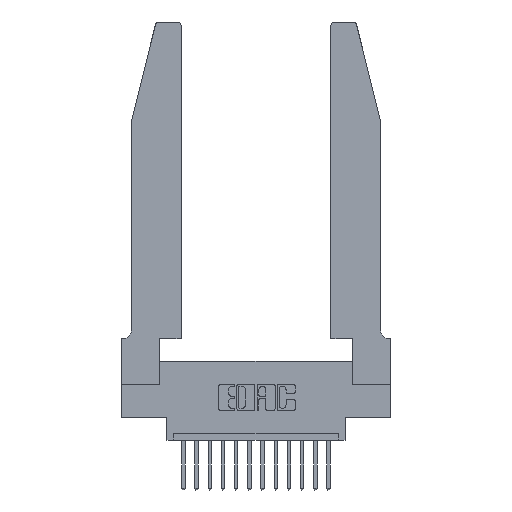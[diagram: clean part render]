
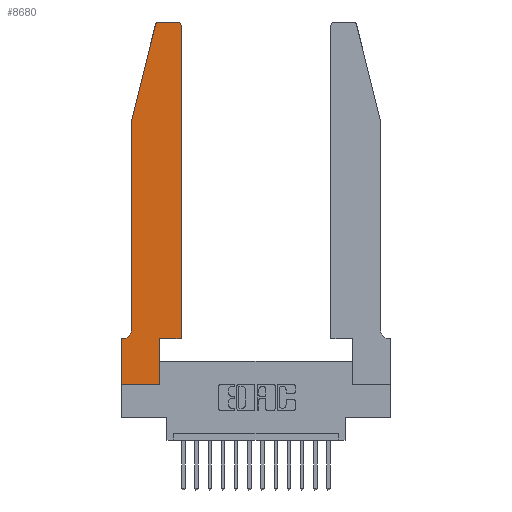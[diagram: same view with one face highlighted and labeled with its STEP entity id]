
A CAD part, top view. The second image highlights one B-rep face of the part: STEP entity #8680.
In plain terms, the highlighted planar face has unit normal (0, 0, 1).
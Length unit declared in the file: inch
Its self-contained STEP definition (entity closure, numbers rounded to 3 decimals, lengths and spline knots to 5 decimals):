
#162 = CARTESIAN_POINT ( 'NONE',  ( 0.0755, 2., 0.37 ) ) ;
#264 = VERTEX_POINT ( 'NONE', #16240 ) ;
#308 = VERTEX_POINT ( 'NONE', #8545 ) ;
#550 = ORIENTED_EDGE ( 'NONE', *, *, #2404, .T. ) ;
#979 = ORIENTED_EDGE ( 'NONE', *, *, #16185, .T. ) ;
#1325 = ORIENTED_EDGE ( 'NONE', *, *, #13754, .T. ) ;
#1422 = EDGE_CURVE ( 'NONE', #3735, #16427, #5521, .T. ) ;
#1451 = ORIENTED_EDGE ( 'NONE', *, *, #1422, .T. ) ;
#1452 = EDGE_CURVE ( 'NONE', #264, #11926, #15490, .T. ) ;
#1501 = CARTESIAN_POINT ( 'NONE',  ( 0.2865, 0.35, 0.37 ) ) ;
#2404 = EDGE_CURVE ( 'NONE', #3888, #9783, #6743, .T. ) ;
#2484 = ORIENTED_EDGE ( 'NONE', *, *, #10499, .T. ) ;
#2509 = LINE ( 'NONE', #3486, #11164 ) ;
#2573 = LINE ( 'NONE', #11310, #11211 ) ;
#2923 = FACE_OUTER_BOUND ( 'NONE', #5593, .T. ) ;
#3100 = EDGE_CURVE ( 'NONE', #11926, #308, #15643, .T. ) ;
#3486 = CARTESIAN_POINT ( 'NONE',  ( 0.4505, 0.35, 0.37 ) ) ;
#3735 = VERTEX_POINT ( 'NONE', #7786 ) ;
#3888 = VERTEX_POINT ( 'NONE', #14912 ) ;
#4211 = DIRECTION ( 'NONE',  ( 0., 1., 0. ) ) ;
#4612 = CARTESIAN_POINT ( 'NONE',  ( 0.284, 2.72, 0.37 ) ) ;
#4702 = AXIS2_PLACEMENT_3D ( 'NONE', #14642, #4958, #8981 ) ;
#4728 = DIRECTION ( 'NONE',  ( 0., 0., 1. ) ) ;
#4818 = VECTOR ( 'NONE', #17328, 39.37008 ) ;
#4958 = DIRECTION ( 'NONE',  ( 0., 0., 1. ) ) ;
#5153 = ORIENTED_EDGE ( 'NONE', *, *, #14551, .T. ) ;
#5156 = VECTOR ( 'NONE', #14626, 39.37008 ) ;
#5386 = DIRECTION ( 'NONE',  ( 0., 1., 0. ) ) ;
#5521 = CIRCLE ( 'NONE', #15368, 0.07 ) ;
#5593 = EDGE_LOOP ( 'NONE', ( #14481, #550, #979, #6981, #1451, #1325, #8827, #8383, #16617, #17822, #2484, #5153 ) ) ;
#5652 = DIRECTION ( 'NONE',  ( -0.239, -0.971, 0. ) ) ;
#6368 = EDGE_CURVE ( 'NONE', #11910, #3888, #15338, .T. ) ;
#6524 = LINE ( 'NONE', #162, #13690 ) ;
#6528 = VERTEX_POINT ( 'NONE', #7620 ) ;
#6743 = CIRCLE ( 'NONE', #10587, 0.03 ) ;
#6981 = ORIENTED_EDGE ( 'NONE', *, *, #10086, .T. ) ;
#7280 = VECTOR ( 'NONE', #5652, 39.37008 ) ;
#7620 = CARTESIAN_POINT ( 'NONE',  ( 0.4505, 0.35, 0.37 ) ) ;
#7624 = EDGE_CURVE ( 'NONE', #9199, #6528, #2509, .T. ) ;
#7756 = CARTESIAN_POINT ( 'NONE',  ( 0.2605, 2.75, 0.37 ) ) ;
#7786 = CARTESIAN_POINT ( 'NONE',  ( 0.0755, 0.42, 0.37 ) ) ;
#7881 = VECTOR ( 'NONE', #5386, 39.37008 ) ;
#7980 = VERTEX_POINT ( 'NONE', #9701 ) ;
#8259 = CARTESIAN_POINT ( 'NONE',  ( 0., 0., 0.37 ) ) ;
#8383 = ORIENTED_EDGE ( 'NONE', *, *, #3100, .T. ) ;
#8545 = CARTESIAN_POINT ( 'NONE',  ( 0.2865, 0., 0.37 ) ) ;
#8680 = ADVANCED_FACE ( 'NONE', ( #2923 ), #17317, .T. ) ;
#8827 = ORIENTED_EDGE ( 'NONE', *, *, #1452, .T. ) ;
#8897 = VERTEX_POINT ( 'NONE', #13616 ) ;
#8981 = DIRECTION ( 'NONE',  ( 1., 0., 0. ) ) ;
#9169 = LINE ( 'NONE', #16476, #7881 ) ;
#9199 = VERTEX_POINT ( 'NONE', #1501 ) ;
#9495 = CIRCLE ( 'NONE', #4702, 0.03 ) ;
#9701 = CARTESIAN_POINT ( 'NONE',  ( 0.4505, 2.72, 0.37 ) ) ;
#9712 = CARTESIAN_POINT ( 'NONE',  ( 0.0755, 2., 0.37 ) ) ;
#9753 = DIRECTION ( 'NONE',  ( -1., 0., 0. ) ) ;
#9783 = VERTEX_POINT ( 'NONE', #9856 ) ;
#9856 = CARTESIAN_POINT ( 'NONE',  ( 0.25487, 2.72718, 0.37 ) ) ;
#10086 = EDGE_CURVE ( 'NONE', #8897, #3735, #6524, .T. ) ;
#10265 = CARTESIAN_POINT ( 'NONE',  ( 0.0055, 0.35, 0.37 ) ) ;
#10380 = CARTESIAN_POINT ( 'NONE',  ( 0., 0., 0.37 ) ) ;
#10499 = EDGE_CURVE ( 'NONE', #6528, #7980, #9169, .T. ) ;
#10552 = AXIS2_PLACEMENT_3D ( 'NONE', #16009, #17997, #16654 ) ;
#10587 = AXIS2_PLACEMENT_3D ( 'NONE', #4612, #4728, #15564 ) ;
#10719 = CARTESIAN_POINT ( 'NONE',  ( 0., 0., 0.37 ) ) ;
#11164 = VECTOR ( 'NONE', #13161, 39.37008 ) ;
#11211 = VECTOR ( 'NONE', #4211, 39.37008 ) ;
#11239 = LINE ( 'NONE', #17971, #17152 ) ;
#11310 = CARTESIAN_POINT ( 'NONE',  ( 0.2865, 0.35, 0.37 ) ) ;
#11381 = DIRECTION ( 'NONE',  ( 0., -1., 0. ) ) ;
#11910 = VERTEX_POINT ( 'NONE', #15789 ) ;
#11926 = VERTEX_POINT ( 'NONE', #10719 ) ;
#12294 = DIRECTION ( 'NONE',  ( -1., 0., 0. ) ) ;
#12614 = DIRECTION ( 'NONE',  ( 0., 0., -1. ) ) ;
#13161 = DIRECTION ( 'NONE',  ( 1., 0., 0. ) ) ;
#13616 = CARTESIAN_POINT ( 'NONE',  ( 0.0755, 2., 0.37 ) ) ;
#13690 = VECTOR ( 'NONE', #15449, 39.37008 ) ;
#13754 = EDGE_CURVE ( 'NONE', #16427, #264, #11239, .T. ) ;
#14481 = ORIENTED_EDGE ( 'NONE', *, *, #6368, .T. ) ;
#14551 = EDGE_CURVE ( 'NONE', #7980, #11910, #9495, .T. ) ;
#14626 = DIRECTION ( 'NONE',  ( -1., 0., 0. ) ) ;
#14642 = CARTESIAN_POINT ( 'NONE',  ( 0.4205, 2.72, 0.37 ) ) ;
#14880 = CARTESIAN_POINT ( 'NONE',  ( 0.0055, 0.42, 0.37 ) ) ;
#14912 = CARTESIAN_POINT ( 'NONE',  ( 0.284, 2.75, 0.37 ) ) ;
#14986 = EDGE_CURVE ( 'NONE', #308, #9199, #2573, .T. ) ;
#15338 = LINE ( 'NONE', #7756, #5156 ) ;
#15368 = AXIS2_PLACEMENT_3D ( 'NONE', #14880, #12614, #9753 ) ;
#15449 = DIRECTION ( 'NONE',  ( 0., -1., 0. ) ) ;
#15490 = LINE ( 'NONE', #8259, #16806 ) ;
#15564 = DIRECTION ( 'NONE',  ( 1., 0., 0. ) ) ;
#15643 = LINE ( 'NONE', #10380, #4818 ) ;
#15789 = CARTESIAN_POINT ( 'NONE',  ( 0.4205, 2.75, 0.37 ) ) ;
#16009 = CARTESIAN_POINT ( 'NONE',  ( 0., 0.35, 0.37 ) ) ;
#16185 = EDGE_CURVE ( 'NONE', #9783, #8897, #17538, .T. ) ;
#16240 = CARTESIAN_POINT ( 'NONE',  ( 0., 0.35, 0.37 ) ) ;
#16427 = VERTEX_POINT ( 'NONE', #10265 ) ;
#16476 = CARTESIAN_POINT ( 'NONE',  ( 0.4505, 0.35, 0.37 ) ) ;
#16617 = ORIENTED_EDGE ( 'NONE', *, *, #14986, .T. ) ;
#16654 = DIRECTION ( 'NONE',  ( 1., 0., 0. ) ) ;
#16806 = VECTOR ( 'NONE', #11381, 39.37008 ) ;
#17152 = VECTOR ( 'NONE', #12294, 39.37008 ) ;
#17317 = PLANE ( 'NONE',  #10552 ) ;
#17328 = DIRECTION ( 'NONE',  ( 1., 0., 0. ) ) ;
#17538 = LINE ( 'NONE', #9712, #7280 ) ;
#17822 = ORIENTED_EDGE ( 'NONE', *, *, #7624, .T. ) ;
#17971 = CARTESIAN_POINT ( 'NONE',  ( 0.0755, 0.35, 0.37 ) ) ;
#17997 = DIRECTION ( 'NONE',  ( 0., 0., 1. ) ) ;
